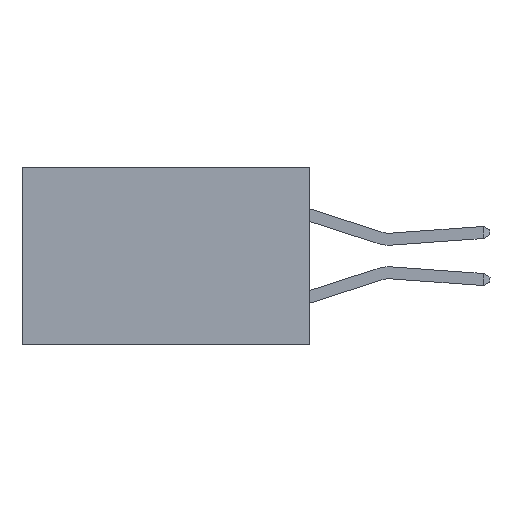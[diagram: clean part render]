
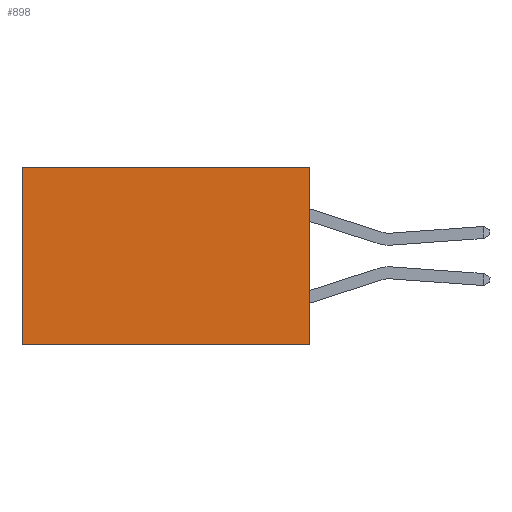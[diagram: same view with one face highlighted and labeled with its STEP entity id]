
A CAD part, left-side view. The second image highlights one B-rep face of the part: STEP entity #898.
In plain terms, the highlighted planar face has unit normal (-1, 0, 0).
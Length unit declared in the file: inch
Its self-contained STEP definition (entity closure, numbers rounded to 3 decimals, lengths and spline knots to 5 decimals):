
#429 = ORIENTED_EDGE ( 'NONE', *, *, #5171, .F. ) ;
#898 = ADVANCED_FACE ( 'NONE', ( #8767 ), #20576, .F. ) ;
#2864 = DIRECTION ( 'NONE',  ( 0., 1., 0. ) ) ;
#3427 = AXIS2_PLACEMENT_3D ( 'NONE', #22967, #20549, #20519 ) ;
#4853 = CARTESIAN_POINT ( 'NONE',  ( 0.2615, 0., 0. ) ) ;
#5171 = EDGE_CURVE ( 'NONE', #22082, #10202, #22655, .T. ) ;
#5211 = DIRECTION ( 'NONE',  ( 0., 1., 0. ) ) ;
#6035 = VERTEX_POINT ( 'NONE', #18980 ) ;
#6041 = VECTOR ( 'NONE', #2864, 39.37008 ) ;
#6557 = CARTESIAN_POINT ( 'NONE',  ( 0.2615, 0.6, -0.37 ) ) ;
#7315 = VECTOR ( 'NONE', #20118, 39.37008 ) ;
#8528 = EDGE_CURVE ( 'NONE', #10202, #13586, #18322, .T. ) ;
#8767 = FACE_OUTER_BOUND ( 'NONE', #18388, .T. ) ;
#10202 = VERTEX_POINT ( 'NONE', #21916 ) ;
#11999 = VECTOR ( 'NONE', #5211, 39.37008 ) ;
#13586 = VERTEX_POINT ( 'NONE', #6557 ) ;
#14666 = DIRECTION ( 'NONE',  ( 0., 0., -1. ) ) ;
#14997 = ORIENTED_EDGE ( 'NONE', *, *, #20619, .T. ) ;
#15863 = VECTOR ( 'NONE', #14666, 39.37008 ) ;
#16332 = CARTESIAN_POINT ( 'NONE',  ( 0.2615, 0., -0.37 ) ) ;
#16779 = CARTESIAN_POINT ( 'NONE',  ( 0.2615, 0., -0.37 ) ) ;
#17493 = EDGE_CURVE ( 'NONE', #6035, #13586, #20983, .T. ) ;
#18322 = LINE ( 'NONE', #16779, #11999 ) ;
#18388 = EDGE_LOOP ( 'NONE', ( #23863, #19905, #429, #14997 ) ) ;
#18980 = CARTESIAN_POINT ( 'NONE',  ( 0.2615, 0.6, 0. ) ) ;
#19905 = ORIENTED_EDGE ( 'NONE', *, *, #8528, .F. ) ;
#20118 = DIRECTION ( 'NONE',  ( 0., 0., -1. ) ) ;
#20519 = DIRECTION ( 'NONE',  ( 0., 0., -1. ) ) ;
#20549 = DIRECTION ( 'NONE',  ( 1., 0., 0. ) ) ;
#20576 = PLANE ( 'NONE',  #3427 ) ;
#20619 = EDGE_CURVE ( 'NONE', #22082, #6035, #21445, .T. ) ;
#20983 = LINE ( 'NONE', #24216, #15863 ) ;
#21345 = CARTESIAN_POINT ( 'NONE',  ( 0.2615, 0., 0. ) ) ;
#21445 = LINE ( 'NONE', #4853, #6041 ) ;
#21916 = CARTESIAN_POINT ( 'NONE',  ( 0.2615, 0., -0.37 ) ) ;
#22082 = VERTEX_POINT ( 'NONE', #21345 ) ;
#22655 = LINE ( 'NONE', #16332, #7315 ) ;
#22967 = CARTESIAN_POINT ( 'NONE',  ( 0.2615, 0., -0.37 ) ) ;
#23863 = ORIENTED_EDGE ( 'NONE', *, *, #17493, .T. ) ;
#24216 = CARTESIAN_POINT ( 'NONE',  ( 0.2615, 0.6, -0.37 ) ) ;
